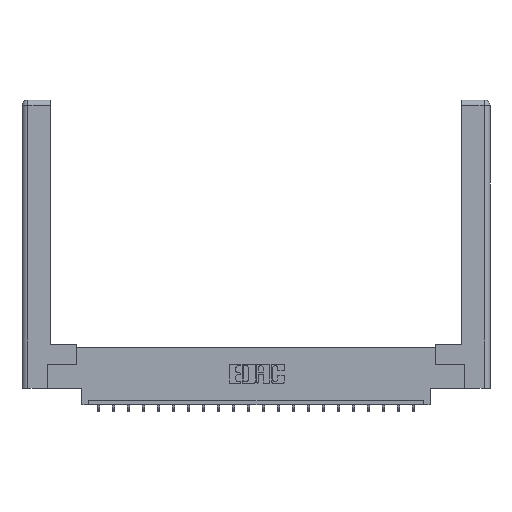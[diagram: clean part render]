
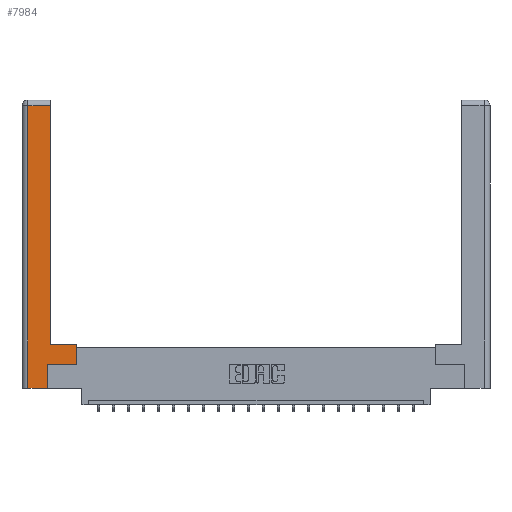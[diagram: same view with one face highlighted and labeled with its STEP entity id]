
A CAD part, top view. The second image highlights one B-rep face of the part: STEP entity #7984.
In plain terms, the highlighted planar face has unit normal (0, 0, 1).
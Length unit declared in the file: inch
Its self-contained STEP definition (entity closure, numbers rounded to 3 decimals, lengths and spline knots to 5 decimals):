
#218 = VERTEX_POINT ( 'NONE', #19512 ) ;
#432 = VECTOR ( 'NONE', #3751, 39.37008 ) ;
#785 = CARTESIAN_POINT ( 'NONE',  ( 0.565, 0.245, 0. ) ) ;
#889 = VERTEX_POINT ( 'NONE', #14027 ) ;
#1087 = LINE ( 'NONE', #16956, #16097 ) ;
#1219 = EDGE_CURVE ( 'NONE', #889, #15437, #15273, .T. ) ;
#1525 = VECTOR ( 'NONE', #9045, 39.37008 ) ;
#2316 = CARTESIAN_POINT ( 'NONE',  ( 0.0615, 0., 0. ) ) ;
#2599 = LINE ( 'NONE', #785, #1525 ) ;
#3348 = CARTESIAN_POINT ( 'NONE',  ( 0.295, 0.45, 0. ) ) ;
#3685 = DIRECTION ( 'NONE',  ( 0., 0., -1. ) ) ;
#3692 = EDGE_CURVE ( 'NONE', #4249, #17188, #7530, .T. ) ;
#3751 = DIRECTION ( 'NONE',  ( 0., 1., 0. ) ) ;
#3869 = VERTEX_POINT ( 'NONE', #21598 ) ;
#4056 = EDGE_CURVE ( 'NONE', #15437, #3869, #1087, .T. ) ;
#4209 = CARTESIAN_POINT ( 'NONE',  ( 0.295, 2.94, 0. ) ) ;
#4249 = VERTEX_POINT ( 'NONE', #20833 ) ;
#4340 = LINE ( 'NONE', #3348, #9860 ) ;
#5213 = DIRECTION ( 'NONE',  ( -1., 0., 0. ) ) ;
#5402 = CARTESIAN_POINT ( 'NONE',  ( 0.565, 0.45, 0. ) ) ;
#5410 = ORIENTED_EDGE ( 'NONE', *, *, #1219, .T. ) ;
#5894 = ORIENTED_EDGE ( 'NONE', *, *, #16380, .T. ) ;
#6124 = AXIS2_PLACEMENT_3D ( 'NONE', #15307, #3685, #5213 ) ;
#6454 = VECTOR ( 'NONE', #18674, 39.37008 ) ;
#6953 = DIRECTION ( 'NONE',  ( 1., 0., 0. ) ) ;
#7261 = FACE_OUTER_BOUND ( 'NONE', #18768, .T. ) ;
#7530 = LINE ( 'NONE', #19065, #432 ) ;
#7984 = ADVANCED_FACE ( 'NONE', ( #7261 ), #18627, .F. ) ;
#8099 = ORIENTED_EDGE ( 'NONE', *, *, #11611, .T. ) ;
#8350 = VECTOR ( 'NONE', #15978, 39.37008 ) ;
#8640 = CARTESIAN_POINT ( 'NONE',  ( 0.565, 0.245, 0. ) ) ;
#9045 = DIRECTION ( 'NONE',  ( 1., 0., 0. ) ) ;
#9860 = VECTOR ( 'NONE', #21666, 39.37008 ) ;
#9864 = LINE ( 'NONE', #5402, #6454 ) ;
#10044 = CARTESIAN_POINT ( 'NONE',  ( 0.0615, 0., 0. ) ) ;
#11016 = LINE ( 'NONE', #14960, #16545 ) ;
#11273 = DIRECTION ( 'NONE',  ( -1., 0., 0. ) ) ;
#11611 = EDGE_CURVE ( 'NONE', #17188, #889, #11016, .T. ) ;
#13298 = VERTEX_POINT ( 'NONE', #13503 ) ;
#13379 = VERTEX_POINT ( 'NONE', #8640 ) ;
#13503 = CARTESIAN_POINT ( 'NONE',  ( 0.565, 0.45, 0. ) ) ;
#13581 = ORIENTED_EDGE ( 'NONE', *, *, #14870, .T. ) ;
#13676 = VECTOR ( 'NONE', #21815, 39.37008 ) ;
#14027 = CARTESIAN_POINT ( 'NONE',  ( 0.0615, 2.94, 0. ) ) ;
#14657 = CARTESIAN_POINT ( 'NONE',  ( 0.265, 0.245, 0. ) ) ;
#14870 = EDGE_CURVE ( 'NONE', #218, #13379, #2599, .T. ) ;
#14960 = CARTESIAN_POINT ( 'NONE',  ( 0.0615, 2.94, 0. ) ) ;
#15273 = LINE ( 'NONE', #10044, #13676 ) ;
#15307 = CARTESIAN_POINT ( 'NONE',  ( 0., 0., 0. ) ) ;
#15437 = VERTEX_POINT ( 'NONE', #2316 ) ;
#15711 = LINE ( 'NONE', #14657, #8350 ) ;
#15978 = DIRECTION ( 'NONE',  ( 0., 1., 0. ) ) ;
#16097 = VECTOR ( 'NONE', #6953, 39.37008 ) ;
#16380 = EDGE_CURVE ( 'NONE', #13379, #13298, #9864, .T. ) ;
#16545 = VECTOR ( 'NONE', #11273, 39.37008 ) ;
#16700 = ORIENTED_EDGE ( 'NONE', *, *, #4056, .T. ) ;
#16956 = CARTESIAN_POINT ( 'NONE',  ( 0.265, 0., 0. ) ) ;
#17188 = VERTEX_POINT ( 'NONE', #4209 ) ;
#17263 = ORIENTED_EDGE ( 'NONE', *, *, #21071, .T. ) ;
#17326 = ORIENTED_EDGE ( 'NONE', *, *, #19559, .T. ) ;
#18627 = PLANE ( 'NONE',  #6124 ) ;
#18674 = DIRECTION ( 'NONE',  ( 0., 1., 0. ) ) ;
#18768 = EDGE_LOOP ( 'NONE', ( #19606, #8099, #5410, #16700, #17326, #13581, #5894, #17263 ) ) ;
#19065 = CARTESIAN_POINT ( 'NONE',  ( 0.295, 3., 0. ) ) ;
#19512 = CARTESIAN_POINT ( 'NONE',  ( 0.265, 0.245, 0. ) ) ;
#19559 = EDGE_CURVE ( 'NONE', #3869, #218, #15711, .T. ) ;
#19606 = ORIENTED_EDGE ( 'NONE', *, *, #3692, .T. ) ;
#20833 = CARTESIAN_POINT ( 'NONE',  ( 0.295, 0.45, 0. ) ) ;
#21071 = EDGE_CURVE ( 'NONE', #13298, #4249, #4340, .T. ) ;
#21598 = CARTESIAN_POINT ( 'NONE',  ( 0.265, 0., 0. ) ) ;
#21666 = DIRECTION ( 'NONE',  ( -1., 0., 0. ) ) ;
#21815 = DIRECTION ( 'NONE',  ( 0., -1., 0. ) ) ;
